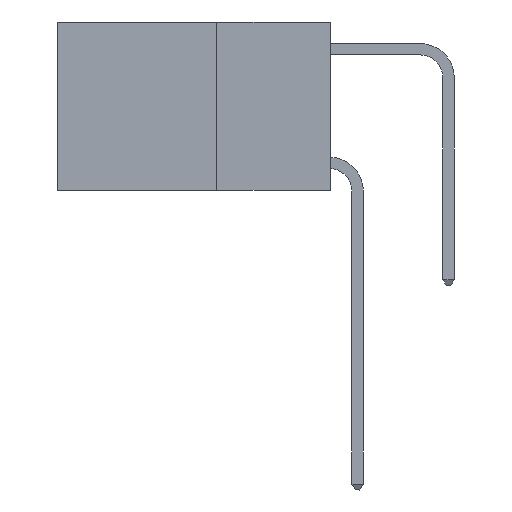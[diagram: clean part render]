
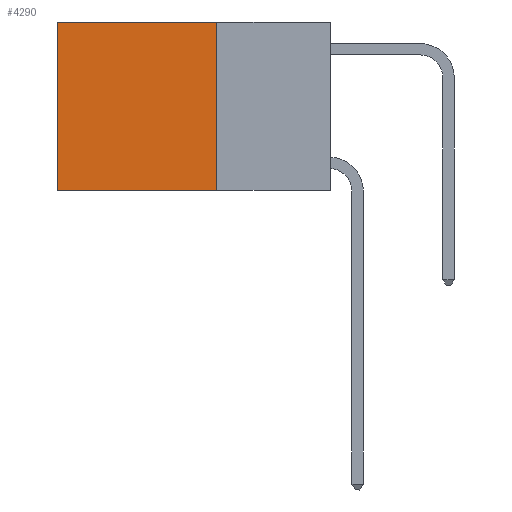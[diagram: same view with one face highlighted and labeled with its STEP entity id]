
A CAD part, left-side view. The second image highlights one B-rep face of the part: STEP entity #4290.
In plain terms, the highlighted planar face has unit normal (-1, 0, 0).
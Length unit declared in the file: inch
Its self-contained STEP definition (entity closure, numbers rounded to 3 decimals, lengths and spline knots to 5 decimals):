
#487 = CARTESIAN_POINT ( 'NONE',  ( 0.2625, 0.25, 0. ) ) ;
#868 = PLANE ( 'NONE',  #13193 ) ;
#1093 = LINE ( 'NONE', #13479, #5690 ) ;
#1154 = VECTOR ( 'NONE', #4554, 39.37008 ) ;
#2249 = CARTESIAN_POINT ( 'NONE',  ( 0.2625, 0.6, -0.37 ) ) ;
#2533 = EDGE_CURVE ( 'NONE', #6406, #5168, #11760, .T. ) ;
#2786 = CARTESIAN_POINT ( 'NONE',  ( 0.2625, 0.6, 0. ) ) ;
#3076 = LINE ( 'NONE', #12333, #10038 ) ;
#3081 = VERTEX_POINT ( 'NONE', #4632 ) ;
#3160 = ORIENTED_EDGE ( 'NONE', *, *, #2533, .T. ) ;
#4234 = DIRECTION ( 'NONE',  ( 0., 0., -1. ) ) ;
#4290 = ADVANCED_FACE ( 'NONE', ( #13448 ), #868, .F. ) ;
#4554 = DIRECTION ( 'NONE',  ( 0., 1., 0. ) ) ;
#4632 = CARTESIAN_POINT ( 'NONE',  ( 0.2625, 0.25, -0.37 ) ) ;
#5168 = VERTEX_POINT ( 'NONE', #2249 ) ;
#5313 = ORIENTED_EDGE ( 'NONE', *, *, #11818, .F. ) ;
#5690 = VECTOR ( 'NONE', #6382, 39.37008 ) ;
#6156 = DIRECTION ( 'NONE',  ( 1., 0., 0. ) ) ;
#6339 = ORIENTED_EDGE ( 'NONE', *, *, #8705, .F. ) ;
#6382 = DIRECTION ( 'NONE',  ( 0., 0., -1. ) ) ;
#6406 = VERTEX_POINT ( 'NONE', #2786 ) ;
#6523 = LINE ( 'NONE', #6593, #1154 ) ;
#6593 = CARTESIAN_POINT ( 'NONE',  ( 0.2625, 0.25, -0.37 ) ) ;
#8466 = ORIENTED_EDGE ( 'NONE', *, *, #12179, .T. ) ;
#8679 = DIRECTION ( 'NONE',  ( 0., 0., -1. ) ) ;
#8705 = EDGE_CURVE ( 'NONE', #3081, #5168, #6523, .T. ) ;
#9203 = VECTOR ( 'NONE', #8679, 39.37008 ) ;
#9694 = CARTESIAN_POINT ( 'NONE',  ( 0.2625, 0.6, 0. ) ) ;
#10038 = VECTOR ( 'NONE', #13464, 39.37008 ) ;
#10065 = EDGE_LOOP ( 'NONE', ( #3160, #6339, #5313, #8466 ) ) ;
#11365 = CARTESIAN_POINT ( 'NONE',  ( 0.2625, 0.25, 0. ) ) ;
#11760 = LINE ( 'NONE', #9694, #9203 ) ;
#11818 = EDGE_CURVE ( 'NONE', #12692, #3081, #1093, .T. ) ;
#12179 = EDGE_CURVE ( 'NONE', #12692, #6406, #3076, .T. ) ;
#12333 = CARTESIAN_POINT ( 'NONE',  ( 0.2625, 0.25, 0. ) ) ;
#12692 = VERTEX_POINT ( 'NONE', #487 ) ;
#13193 = AXIS2_PLACEMENT_3D ( 'NONE', #11365, #6156, #4234 ) ;
#13448 = FACE_OUTER_BOUND ( 'NONE', #10065, .T. ) ;
#13464 = DIRECTION ( 'NONE',  ( 0., 1., 0. ) ) ;
#13479 = CARTESIAN_POINT ( 'NONE',  ( 0.2625, 0.25, 0. ) ) ;
